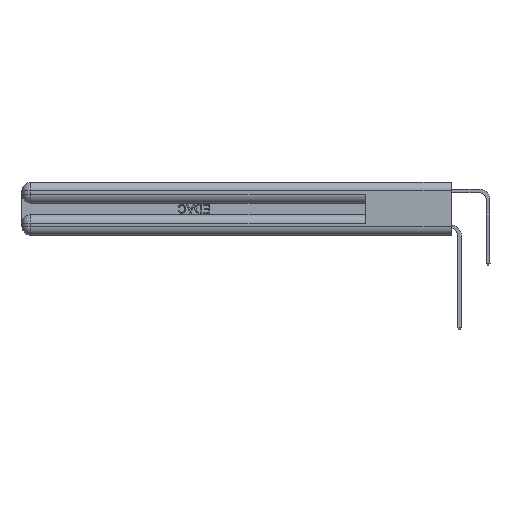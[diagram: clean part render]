
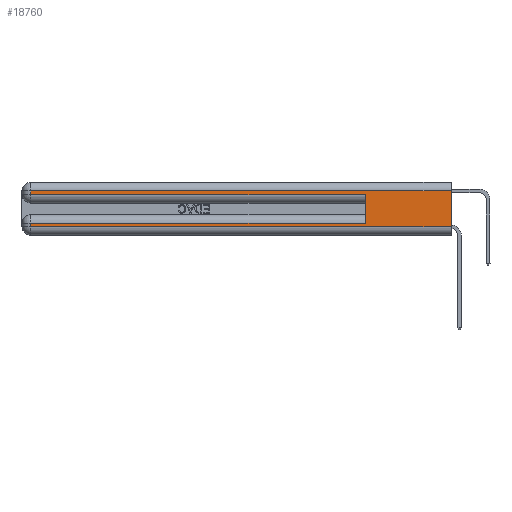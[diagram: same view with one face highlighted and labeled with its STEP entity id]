
A CAD part, left-side view. The second image highlights one B-rep face of the part: STEP entity #18760.
In plain terms, the highlighted planar face has unit normal (-1, 0, 0).
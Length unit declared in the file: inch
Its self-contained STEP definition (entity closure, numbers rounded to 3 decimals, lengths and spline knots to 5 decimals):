
#1 = EDGE_CURVE ( 'NONE', #14547, #4083, #20802, .T. ) ;
#84 = EDGE_CURVE ( 'NONE', #5424, #4083, #1821, .T. ) ;
#136 = LINE ( 'NONE', #2702, #17234 ) ;
#382 = ORIENTED_EDGE ( 'NONE', *, *, #1, .T. ) ;
#454 = DIRECTION ( 'NONE',  ( 0., 1., 0. ) ) ;
#1821 = LINE ( 'NONE', #6181, #9995 ) ;
#2031 = VERTEX_POINT ( 'NONE', #3231 ) ;
#2369 = VERTEX_POINT ( 'NONE', #5165 ) ;
#2702 = CARTESIAN_POINT ( 'NONE',  ( 0., 2.94, 0.37 ) ) ;
#3231 = CARTESIAN_POINT ( 'NONE',  ( 0., 0., 0.31 ) ) ;
#3554 = LINE ( 'NONE', #7554, #20256 ) ;
#4083 = VERTEX_POINT ( 'NONE', #27180 ) ;
#4680 = EDGE_CURVE ( 'NONE', #15418, #30312, #19875, .T. ) ;
#5165 = CARTESIAN_POINT ( 'NONE',  ( 0., 2.94, 0.31 ) ) ;
#5424 = VERTEX_POINT ( 'NONE', #9474 ) ;
#6181 = CARTESIAN_POINT ( 'NONE',  ( 0., 0.6, 0.145 ) ) ;
#7554 = CARTESIAN_POINT ( 'NONE',  ( 0., 0., 0.31 ) ) ;
#7769 = VECTOR ( 'NONE', #10140, 39.37008 ) ;
#8325 = EDGE_CURVE ( 'NONE', #2031, #30312, #22979, .T. ) ;
#8328 = ORIENTED_EDGE ( 'NONE', *, *, #9374, .T. ) ;
#8335 = DIRECTION ( 'NONE',  ( 0., 0., 1. ) ) ;
#8696 = CARTESIAN_POINT ( 'NONE',  ( 0., 0., 0.085 ) ) ;
#8785 = EDGE_CURVE ( 'NONE', #5424, #9566, #17320, .T. ) ;
#9374 = EDGE_CURVE ( 'NONE', #9566, #15418, #20671, .T. ) ;
#9474 = CARTESIAN_POINT ( 'NONE',  ( 0., 0.6, 0.085 ) ) ;
#9566 = VERTEX_POINT ( 'NONE', #28241 ) ;
#9601 = VECTOR ( 'NONE', #18326, 39.37008 ) ;
#9702 = EDGE_LOOP ( 'NONE', ( #27957, #18465, #27358, #382, #25289, #21004, #8328, #24255 ) ) ;
#9995 = VECTOR ( 'NONE', #8335, 39.37008 ) ;
#10140 = DIRECTION ( 'NONE',  ( 0., -1., 0. ) ) ;
#11020 = DIRECTION ( 'NONE',  ( 0., 1., 0. ) ) ;
#12867 = DIRECTION ( 'NONE',  ( 0., 0., -1. ) ) ;
#14547 = VERTEX_POINT ( 'NONE', #17933 ) ;
#14849 = CARTESIAN_POINT ( 'NONE',  ( 0., 0., 0.285 ) ) ;
#15067 = VECTOR ( 'NONE', #11020, 39.37008 ) ;
#15418 = VERTEX_POINT ( 'NONE', #15569 ) ;
#15569 = CARTESIAN_POINT ( 'NONE',  ( 0., 2.94, 0.06 ) ) ;
#17234 = VECTOR ( 'NONE', #29194, 39.37008 ) ;
#17271 = CARTESIAN_POINT ( 'NONE',  ( 0., 0., 0.06 ) ) ;
#17320 = LINE ( 'NONE', #8696, #15067 ) ;
#17933 = CARTESIAN_POINT ( 'NONE',  ( 0., 2.94, 0.285 ) ) ;
#18326 = DIRECTION ( 'NONE',  ( 0., 0., -1. ) ) ;
#18331 = EDGE_CURVE ( 'NONE', #2031, #2369, #3554, .T. ) ;
#18465 = ORIENTED_EDGE ( 'NONE', *, *, #18331, .T. ) ;
#18760 = ADVANCED_FACE ( 'NONE', ( #24738 ), #23233, .F. ) ;
#18930 = EDGE_CURVE ( 'NONE', #2369, #14547, #136, .T. ) ;
#19875 = LINE ( 'NONE', #17271, #30297 ) ;
#20256 = VECTOR ( 'NONE', #454, 39.37008 ) ;
#20671 = LINE ( 'NONE', #22120, #30326 ) ;
#20802 = LINE ( 'NONE', #14849, #7769 ) ;
#21004 = ORIENTED_EDGE ( 'NONE', *, *, #8785, .T. ) ;
#21034 = DIRECTION ( 'NONE',  ( 0., 0., -1. ) ) ;
#22120 = CARTESIAN_POINT ( 'NONE',  ( 0., 2.94, 0.37 ) ) ;
#22979 = LINE ( 'NONE', #30199, #9601 ) ;
#23233 = PLANE ( 'NONE',  #24187 ) ;
#24187 = AXIS2_PLACEMENT_3D ( 'NONE', #30592, #30378, #21034 ) ;
#24255 = ORIENTED_EDGE ( 'NONE', *, *, #4680, .T. ) ;
#24738 = FACE_OUTER_BOUND ( 'NONE', #9702, .T. ) ;
#25289 = ORIENTED_EDGE ( 'NONE', *, *, #84, .F. ) ;
#25395 = CARTESIAN_POINT ( 'NONE',  ( 0., 0., 0.06 ) ) ;
#27180 = CARTESIAN_POINT ( 'NONE',  ( 0., 0.6, 0.285 ) ) ;
#27358 = ORIENTED_EDGE ( 'NONE', *, *, #18930, .T. ) ;
#27957 = ORIENTED_EDGE ( 'NONE', *, *, #8325, .F. ) ;
#28241 = CARTESIAN_POINT ( 'NONE',  ( 0., 2.94, 0.085 ) ) ;
#28958 = DIRECTION ( 'NONE',  ( 0., -1., 0. ) ) ;
#29194 = DIRECTION ( 'NONE',  ( 0., 0., -1. ) ) ;
#30199 = CARTESIAN_POINT ( 'NONE',  ( 0., 0., 0.37 ) ) ;
#30297 = VECTOR ( 'NONE', #28958, 39.37008 ) ;
#30312 = VERTEX_POINT ( 'NONE', #25395 ) ;
#30326 = VECTOR ( 'NONE', #12867, 39.37008 ) ;
#30378 = DIRECTION ( 'NONE',  ( 1., 0., 0. ) ) ;
#30592 = CARTESIAN_POINT ( 'NONE',  ( 0., 0., 0.37 ) ) ;
